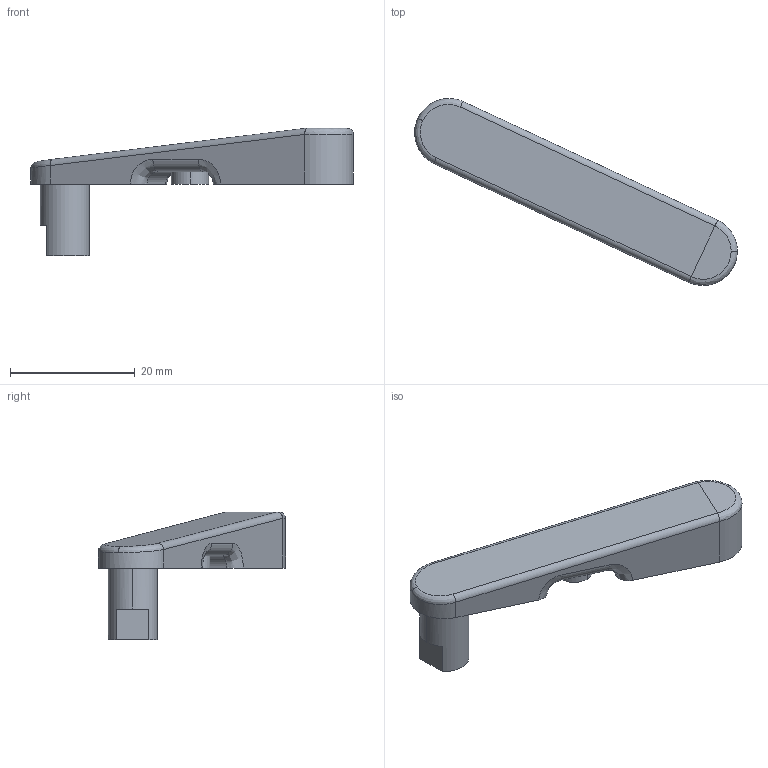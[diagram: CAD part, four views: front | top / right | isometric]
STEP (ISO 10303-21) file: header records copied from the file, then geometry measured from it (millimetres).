
FILE_DESCRIPTION (( 'STEP AP214' ), '1' );
FILE_NAME ('Imura_V2_Release_Lever_Left.step', '2015-01-26T00:08:41', ( 'WarFairy' ), ( '' ), 'SwSTEP 2.0', 'SolidWorks 2013', '' );
FILE_SCHEMA (( 'AUTOMOTIVE_DESIGN' ));
Length unit declared in the file: millimetre
Products named in the file (1): Imura_V2_Release_Lever_Left
Bounding box: 51.78 x 30.01 x 20.5 mm (x, y, z)
Volume: 4128.5 mm3; surface area: 2208.5 mm2
Topology: 1 solids, 1 shells, 33 faces, 79 edges, 50 vertices
Faces by surface type: cylinder 14, plane 11, bspline 8
Entity records: 1338 total; most frequent: CARTESIAN_POINT 596, ORIENTED_EDGE 158, DIRECTION 137, EDGE_CURVE 79, AXIS2_PLACEMENT_3D 53, VERTEX_POINT 50, EDGE_LOOP 35, FACE_OUTER_BOUND 33
